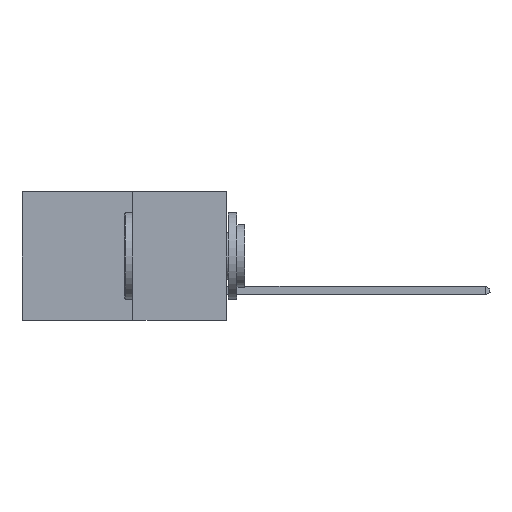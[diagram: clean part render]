
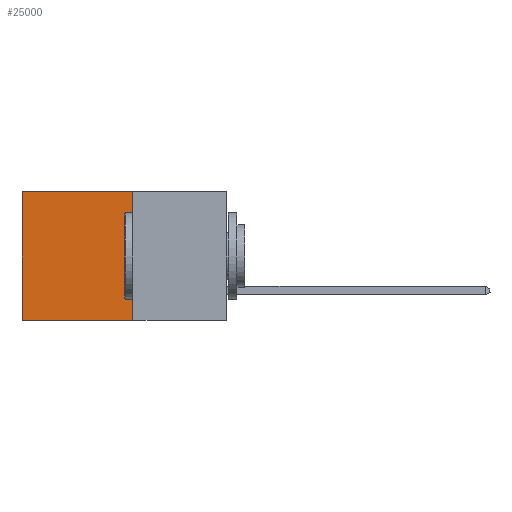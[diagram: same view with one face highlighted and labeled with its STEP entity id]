
A CAD part, left-side view. The second image highlights one B-rep face of the part: STEP entity #25000.
In plain terms, the highlighted planar face has unit normal (-1, 0, 0).
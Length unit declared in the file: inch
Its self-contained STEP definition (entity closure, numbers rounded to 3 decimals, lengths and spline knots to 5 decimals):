
#768 = DIRECTION ( 'NONE',  ( 0., 1., 0. ) ) ;
#932 = VERTEX_POINT ( 'NONE', #10500 ) ;
#1062 = CARTESIAN_POINT ( 'NONE',  ( 0.277, 0.27, -0.37 ) ) ;
#1112 = EDGE_CURVE ( 'NONE', #932, #2718, #16367, .T. ) ;
#1422 = AXIS2_PLACEMENT_3D ( 'NONE', #1062, #13540, #31030 ) ;
#2049 = DIRECTION ( 'NONE',  ( 0., 0., -1. ) ) ;
#2718 = VERTEX_POINT ( 'NONE', #27362 ) ;
#3387 = DIRECTION ( 'NONE',  ( 0., 0., -1. ) ) ;
#3662 = VECTOR ( 'NONE', #2049, 39.37008 ) ;
#3917 = ORIENTED_EDGE ( 'NONE', *, *, #30816, .F. ) ;
#5932 = ORIENTED_EDGE ( 'NONE', *, *, #24670, .T. ) ;
#6314 = DIRECTION ( 'NONE',  ( 0., 1., 0. ) ) ;
#9462 = ORIENTED_EDGE ( 'NONE', *, *, #1112, .F. ) ;
#9864 = ORIENTED_EDGE ( 'NONE', *, *, #12437, .T. ) ;
#10500 = CARTESIAN_POINT ( 'NONE',  ( 0.277, 0.27, -0.37 ) ) ;
#10507 = VERTEX_POINT ( 'NONE', #24361 ) ;
#12158 = EDGE_LOOP ( 'NONE', ( #5932, #9462, #3917, #9864 ) ) ;
#12437 = EDGE_CURVE ( 'NONE', #12895, #10507, #17874, .T. ) ;
#12732 = LINE ( 'NONE', #15803, #31905 ) ;
#12895 = VERTEX_POINT ( 'NONE', #22375 ) ;
#13540 = DIRECTION ( 'NONE',  ( 1., 0., 0. ) ) ;
#14009 = CARTESIAN_POINT ( 'NONE',  ( 0.277, 0.27, -0.37 ) ) ;
#15674 = CARTESIAN_POINT ( 'NONE',  ( 0.277, 0.27, 0. ) ) ;
#15803 = CARTESIAN_POINT ( 'NONE',  ( 0.277, 0.27, -0.37 ) ) ;
#16367 = LINE ( 'NONE', #14009, #29638 ) ;
#16934 = LINE ( 'NONE', #31919, #3662 ) ;
#17874 = LINE ( 'NONE', #15674, #30334 ) ;
#20579 = FACE_OUTER_BOUND ( 'NONE', #12158, .T. ) ;
#22375 = CARTESIAN_POINT ( 'NONE',  ( 0.277, 0.27, 0. ) ) ;
#24361 = CARTESIAN_POINT ( 'NONE',  ( 0.277, 0.59, 0. ) ) ;
#24670 = EDGE_CURVE ( 'NONE', #10507, #2718, #16934, .T. ) ;
#25000 = ADVANCED_FACE ( 'NONE', ( #20579 ), #28538, .F. ) ;
#27362 = CARTESIAN_POINT ( 'NONE',  ( 0.277, 0.59, -0.37 ) ) ;
#28538 = PLANE ( 'NONE',  #1422 ) ;
#29638 = VECTOR ( 'NONE', #6314, 39.37008 ) ;
#30334 = VECTOR ( 'NONE', #768, 39.37008 ) ;
#30816 = EDGE_CURVE ( 'NONE', #12895, #932, #12732, .T. ) ;
#31030 = DIRECTION ( 'NONE',  ( 0., 0., -1. ) ) ;
#31905 = VECTOR ( 'NONE', #3387, 39.37008 ) ;
#31919 = CARTESIAN_POINT ( 'NONE',  ( 0.277, 0.59, -0.37 ) ) ;
